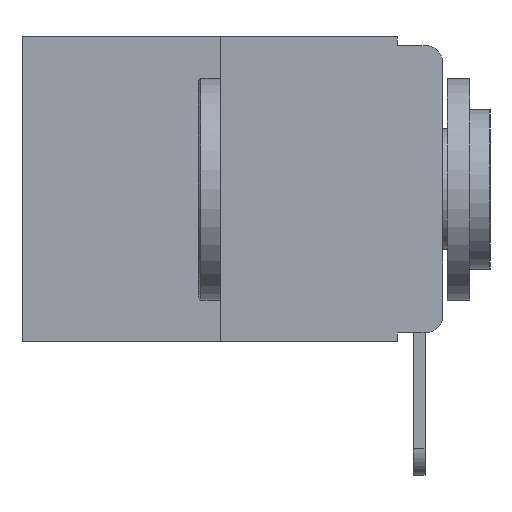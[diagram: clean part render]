
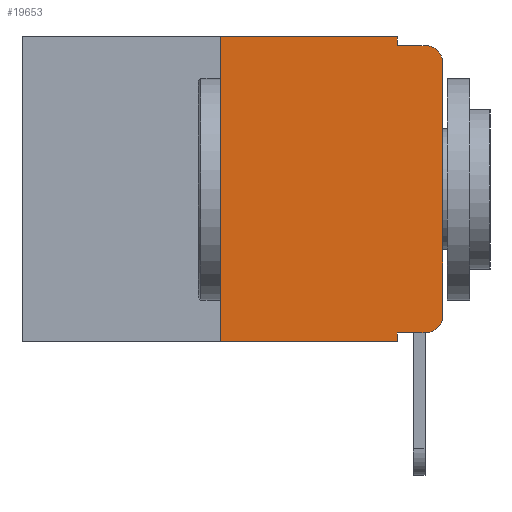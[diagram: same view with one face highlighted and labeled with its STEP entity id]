
A CAD part, left-side view. The second image highlights one B-rep face of the part: STEP entity #19653.
In plain terms, the highlighted planar face has unit normal (-1, 0, 0).
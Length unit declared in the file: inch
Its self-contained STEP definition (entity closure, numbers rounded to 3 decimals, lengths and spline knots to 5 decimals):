
#920 = DIRECTION ( 'NONE',  ( 0., -1., 0. ) ) ;
#1092 = LINE ( 'NONE', #2985, #8989 ) ;
#1663 = VERTEX_POINT ( 'NONE', #12612 ) ;
#1675 = VERTEX_POINT ( 'NONE', #16498 ) ;
#1766 = EDGE_CURVE ( 'NONE', #13356, #1663, #6237, .T. ) ;
#2148 = EDGE_CURVE ( 'NONE', #1675, #6280, #13556, .T. ) ;
#2400 = ORIENTED_EDGE ( 'NONE', *, *, #19522, .F. ) ;
#2850 = DIRECTION ( 'NONE',  ( -1., 0., 0. ) ) ;
#2966 = VERTEX_POINT ( 'NONE', #19437 ) ;
#2985 = CARTESIAN_POINT ( 'NONE',  ( 0., 0.051, -0.01 ) ) ;
#3138 = CARTESIAN_POINT ( 'NONE',  ( 0., 0.051, 0. ) ) ;
#3195 = VERTEX_POINT ( 'NONE', #18548 ) ;
#3201 = ORIENTED_EDGE ( 'NONE', *, *, #2148, .T. ) ;
#3283 = VERTEX_POINT ( 'NONE', #18634 ) ;
#3532 = DIRECTION ( 'NONE',  ( 0., 0., -1. ) ) ;
#3794 = EDGE_CURVE ( 'NONE', #2966, #21292, #9828, .T. ) ;
#3861 = EDGE_CURVE ( 'NONE', #3283, #7492, #15503, .T. ) ;
#3980 = ORIENTED_EDGE ( 'NONE', *, *, #18369, .F. ) ;
#4240 = VECTOR ( 'NONE', #920, 39.37008 ) ;
#4255 = VECTOR ( 'NONE', #13976, 39.37008 ) ;
#4354 = ORIENTED_EDGE ( 'NONE', *, *, #23172, .F. ) ;
#4369 = CARTESIAN_POINT ( 'NONE',  ( 0., 0.051, -0.333 ) ) ;
#4686 = AXIS2_PLACEMENT_3D ( 'NONE', #14085, #12356, #5089 ) ;
#4780 = CARTESIAN_POINT ( 'NONE',  ( 0., 0.051, 0. ) ) ;
#4786 = DIRECTION ( 'NONE',  ( 0., 0., -1. ) ) ;
#5089 = DIRECTION ( 'NONE',  ( 0., 0., -1. ) ) ;
#5616 = CARTESIAN_POINT ( 'NONE',  ( 0., 0.473, -0.343 ) ) ;
#6237 = LINE ( 'NONE', #3138, #21166 ) ;
#6280 = VERTEX_POINT ( 'NONE', #14159 ) ;
#6305 = CARTESIAN_POINT ( 'NONE',  ( 0., 0.02, -0.313 ) ) ;
#6411 = ORIENTED_EDGE ( 'NONE', *, *, #1766, .F. ) ;
#6498 = CARTESIAN_POINT ( 'NONE',  ( 0., 0.473, 0. ) ) ;
#7492 = VERTEX_POINT ( 'NONE', #17636 ) ;
#7647 = ORIENTED_EDGE ( 'NONE', *, *, #21563, .T. ) ;
#8578 = VECTOR ( 'NONE', #14923, 39.37008 ) ;
#8669 = CARTESIAN_POINT ( 'NONE',  ( 0., 0.25, 0. ) ) ;
#8989 = VECTOR ( 'NONE', #15785, 39.37008 ) ;
#9017 = DIRECTION ( 'NONE',  ( 0., 0., 1. ) ) ;
#9754 = CARTESIAN_POINT ( 'NONE',  ( 0., 0., -0.03 ) ) ;
#9828 = LINE ( 'NONE', #21749, #14651 ) ;
#11069 = DIRECTION ( 'NONE',  ( 0., -1., 0. ) ) ;
#12336 = VECTOR ( 'NONE', #3532, 39.37008 ) ;
#12356 = DIRECTION ( 'NONE',  ( 1., 0., 0. ) ) ;
#12538 = EDGE_LOOP ( 'NONE', ( #20583, #7647, #2400, #6411, #3980, #4354, #13920, #14907, #3201, #22894 ) ) ;
#12612 = CARTESIAN_POINT ( 'NONE',  ( 0., 0.051, -0.01 ) ) ;
#12756 = EDGE_CURVE ( 'NONE', #6280, #2966, #13332, .T. ) ;
#13079 = CARTESIAN_POINT ( 'NONE',  ( 0., 0.02, -0.03 ) ) ;
#13161 = CIRCLE ( 'NONE', #14078, 0.02 ) ;
#13332 = CIRCLE ( 'NONE', #15175, 0.02 ) ;
#13356 = VERTEX_POINT ( 'NONE', #4780 ) ;
#13556 = LINE ( 'NONE', #4369, #4240 ) ;
#13643 = LINE ( 'NONE', #14773, #8578 ) ;
#13654 = DIRECTION ( 'NONE',  ( 0., 0., -1. ) ) ;
#13920 = ORIENTED_EDGE ( 'NONE', *, *, #3861, .T. ) ;
#13976 = DIRECTION ( 'NONE',  ( 0., -1., 0. ) ) ;
#14078 = AXIS2_PLACEMENT_3D ( 'NONE', #13079, #20195, #18161 ) ;
#14085 = CARTESIAN_POINT ( 'NONE',  ( 0., 0.473, 0. ) ) ;
#14159 = CARTESIAN_POINT ( 'NONE',  ( 0., 0.02, -0.333 ) ) ;
#14651 = VECTOR ( 'NONE', #9017, 39.37008 ) ;
#14773 = CARTESIAN_POINT ( 'NONE',  ( 0., 0.25, 0. ) ) ;
#14907 = ORIENTED_EDGE ( 'NONE', *, *, #16203, .F. ) ;
#14923 = DIRECTION ( 'NONE',  ( 0., 0., 1. ) ) ;
#15175 = AXIS2_PLACEMENT_3D ( 'NONE', #6305, #2850, #13654 ) ;
#15503 = LINE ( 'NONE', #5616, #17735 ) ;
#15785 = DIRECTION ( 'NONE',  ( 0., -1., 0. ) ) ;
#16203 = EDGE_CURVE ( 'NONE', #1675, #7492, #20189, .T. ) ;
#16498 = CARTESIAN_POINT ( 'NONE',  ( 0., 0.051, -0.333 ) ) ;
#17636 = CARTESIAN_POINT ( 'NONE',  ( 0., 0.051, -0.343 ) ) ;
#17735 = VECTOR ( 'NONE', #11069, 39.37008 ) ;
#17877 = CARTESIAN_POINT ( 'NONE',  ( 0., 0.051, 0. ) ) ;
#17994 = FACE_OUTER_BOUND ( 'NONE', #12538, .T. ) ;
#18161 = DIRECTION ( 'NONE',  ( 0., 0., -1. ) ) ;
#18369 = EDGE_CURVE ( 'NONE', #21326, #13356, #20311, .T. ) ;
#18548 = CARTESIAN_POINT ( 'NONE',  ( 0., 0.02, -0.01 ) ) ;
#18634 = CARTESIAN_POINT ( 'NONE',  ( 0., 0.25, -0.343 ) ) ;
#19437 = CARTESIAN_POINT ( 'NONE',  ( 0., 0., -0.313 ) ) ;
#19522 = EDGE_CURVE ( 'NONE', #1663, #3195, #1092, .T. ) ;
#19653 = ADVANCED_FACE ( 'NONE', ( #17994 ), #21303, .F. ) ;
#20189 = LINE ( 'NONE', #17877, #12336 ) ;
#20195 = DIRECTION ( 'NONE',  ( -1., 0., 0. ) ) ;
#20311 = LINE ( 'NONE', #6498, #4255 ) ;
#20583 = ORIENTED_EDGE ( 'NONE', *, *, #3794, .T. ) ;
#21166 = VECTOR ( 'NONE', #4786, 39.37008 ) ;
#21292 = VERTEX_POINT ( 'NONE', #9754 ) ;
#21303 = PLANE ( 'NONE',  #4686 ) ;
#21326 = VERTEX_POINT ( 'NONE', #8669 ) ;
#21563 = EDGE_CURVE ( 'NONE', #21292, #3195, #13161, .T. ) ;
#21749 = CARTESIAN_POINT ( 'NONE',  ( 0., 0., 0. ) ) ;
#22894 = ORIENTED_EDGE ( 'NONE', *, *, #12756, .T. ) ;
#23172 = EDGE_CURVE ( 'NONE', #3283, #21326, #13643, .T. ) ;
